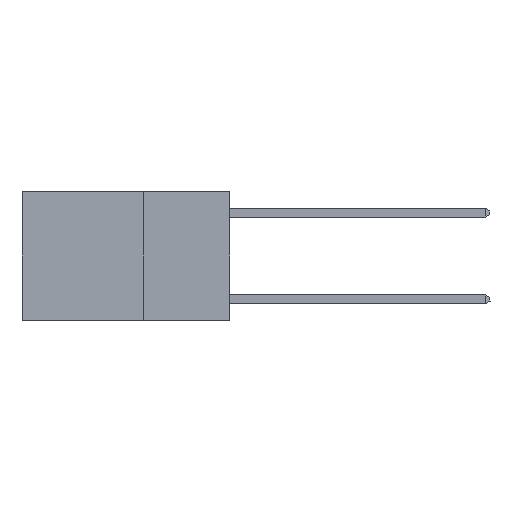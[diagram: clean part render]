
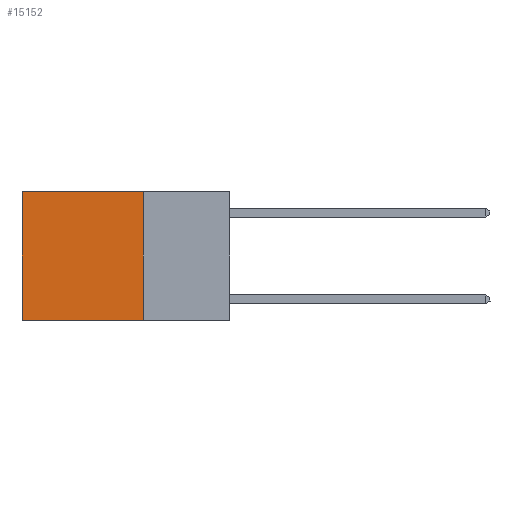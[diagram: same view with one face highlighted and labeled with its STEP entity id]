
A CAD part, left-side view. The second image highlights one B-rep face of the part: STEP entity #15152.
In plain terms, the highlighted planar face has unit normal (-1, 0, 0).
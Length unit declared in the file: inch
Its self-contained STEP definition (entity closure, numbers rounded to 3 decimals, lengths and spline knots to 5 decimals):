
#49 = ORIENTED_EDGE ( 'NONE', *, *, #24161, .F. ) ;
#1025 = VECTOR ( 'NONE', #22794, 39.37008 ) ;
#1038 = CARTESIAN_POINT ( 'NONE',  ( 0.2625, 0.25, -0.37 ) ) ;
#2965 = CARTESIAN_POINT ( 'NONE',  ( 0.2625, 0.6, -0.37 ) ) ;
#4348 = DIRECTION ( 'NONE',  ( 0., 1., 0. ) ) ;
#4889 = ORIENTED_EDGE ( 'NONE', *, *, #17160, .F. ) ;
#5117 = CARTESIAN_POINT ( 'NONE',  ( 0.2625, 0.25, 0. ) ) ;
#5560 = VECTOR ( 'NONE', #4348, 39.37008 ) ;
#6523 = LINE ( 'NONE', #20755, #1025 ) ;
#6780 = LINE ( 'NONE', #5117, #22431 ) ;
#7486 = DIRECTION ( 'NONE',  ( 0., 0., -1. ) ) ;
#8175 = EDGE_CURVE ( 'NONE', #9997, #17132, #6523, .T. ) ;
#8220 = FACE_OUTER_BOUND ( 'NONE', #12977, .T. ) ;
#8310 = AXIS2_PLACEMENT_3D ( 'NONE', #15648, #19738, #7486 ) ;
#9011 = VECTOR ( 'NONE', #13385, 39.37008 ) ;
#9272 = DIRECTION ( 'NONE',  ( 0., 0., -1. ) ) ;
#9997 = VERTEX_POINT ( 'NONE', #15446 ) ;
#12977 = EDGE_LOOP ( 'NONE', ( #15810, #49, #4889, #18682 ) ) ;
#13385 = DIRECTION ( 'NONE',  ( 0., 1., 0. ) ) ;
#13580 = PLANE ( 'NONE',  #8310 ) ;
#13742 = VERTEX_POINT ( 'NONE', #25734 ) ;
#13820 = LINE ( 'NONE', #1038, #9011 ) ;
#14600 = CARTESIAN_POINT ( 'NONE',  ( 0.2625, 0.25, 0. ) ) ;
#15152 = ADVANCED_FACE ( 'NONE', ( #8220 ), #13580, .F. ) ;
#15446 = CARTESIAN_POINT ( 'NONE',  ( 0.2625, 0.6, 0. ) ) ;
#15648 = CARTESIAN_POINT ( 'NONE',  ( 0.2625, 0.25, 0. ) ) ;
#15810 = ORIENTED_EDGE ( 'NONE', *, *, #8175, .T. ) ;
#16197 = EDGE_CURVE ( 'NONE', #21282, #9997, #21872, .T. ) ;
#17132 = VERTEX_POINT ( 'NONE', #2965 ) ;
#17160 = EDGE_CURVE ( 'NONE', #21282, #13742, #6780, .T. ) ;
#18682 = ORIENTED_EDGE ( 'NONE', *, *, #16197, .T. ) ;
#19738 = DIRECTION ( 'NONE',  ( 1., 0., 0. ) ) ;
#20358 = CARTESIAN_POINT ( 'NONE',  ( 0.2625, 0.25, 0. ) ) ;
#20755 = CARTESIAN_POINT ( 'NONE',  ( 0.2625, 0.6, 0. ) ) ;
#21282 = VERTEX_POINT ( 'NONE', #20358 ) ;
#21872 = LINE ( 'NONE', #14600, #5560 ) ;
#22431 = VECTOR ( 'NONE', #9272, 39.37008 ) ;
#22794 = DIRECTION ( 'NONE',  ( 0., 0., -1. ) ) ;
#24161 = EDGE_CURVE ( 'NONE', #13742, #17132, #13820, .T. ) ;
#25734 = CARTESIAN_POINT ( 'NONE',  ( 0.2625, 0.25, -0.37 ) ) ;
